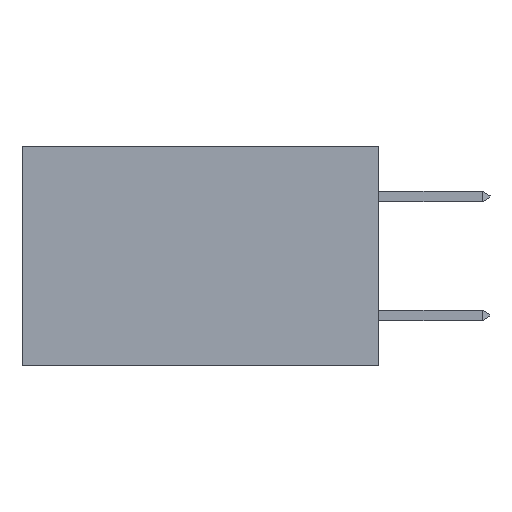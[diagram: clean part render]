
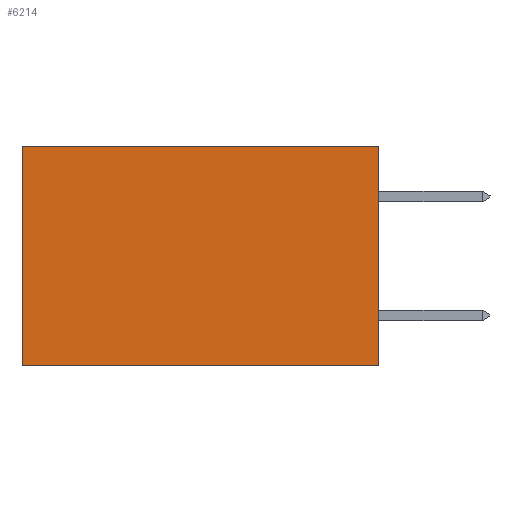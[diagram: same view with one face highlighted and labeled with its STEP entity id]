
A CAD part, left-side view. The second image highlights one B-rep face of the part: STEP entity #6214.
In plain terms, the highlighted planar face has unit normal (-1, 0, 0).
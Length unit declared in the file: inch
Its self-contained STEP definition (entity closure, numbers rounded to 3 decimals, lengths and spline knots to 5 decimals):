
#232 = DIRECTION ( 'NONE',  ( 0., 0., -1. ) ) ;
#414 = VERTEX_POINT ( 'NONE', #10315 ) ;
#859 = DIRECTION ( 'NONE',  ( 0., 1., 0. ) ) ;
#1289 = CARTESIAN_POINT ( 'NONE',  ( 0.2615, 0., 0. ) ) ;
#2617 = CARTESIAN_POINT ( 'NONE',  ( 0.2615, 0.6, -0.37 ) ) ;
#3015 = LINE ( 'NONE', #9256, #19265 ) ;
#3797 = AXIS2_PLACEMENT_3D ( 'NONE', #9443, #17130, #232 ) ;
#4141 = EDGE_CURVE ( 'NONE', #414, #11413, #12224, .T. ) ;
#4582 = EDGE_CURVE ( 'NONE', #12774, #414, #8636, .T. ) ;
#5208 = DIRECTION ( 'NONE',  ( 0., 0., -1. ) ) ;
#5294 = ORIENTED_EDGE ( 'NONE', *, *, #4582, .T. ) ;
#5436 = VECTOR ( 'NONE', #5208, 39.37008 ) ;
#5633 = ORIENTED_EDGE ( 'NONE', *, *, #19944, .F. ) ;
#5884 = DIRECTION ( 'NONE',  ( 0., 0., -1. ) ) ;
#5944 = VECTOR ( 'NONE', #859, 39.37008 ) ;
#6214 = ADVANCED_FACE ( 'NONE', ( #8006 ), #14265, .F. ) ;
#8006 = FACE_OUTER_BOUND ( 'NONE', #9538, .T. ) ;
#8281 = LINE ( 'NONE', #19129, #5436 ) ;
#8636 = LINE ( 'NONE', #19574, #5944 ) ;
#8800 = EDGE_CURVE ( 'NONE', #12774, #17832, #8281, .T. ) ;
#9256 = CARTESIAN_POINT ( 'NONE',  ( 0.2615, 0., -0.37 ) ) ;
#9443 = CARTESIAN_POINT ( 'NONE',  ( 0.2615, 0., -0.37 ) ) ;
#9538 = EDGE_LOOP ( 'NONE', ( #17155, #5633, #17065, #5294 ) ) ;
#10152 = CARTESIAN_POINT ( 'NONE',  ( 0.2615, 0., -0.37 ) ) ;
#10315 = CARTESIAN_POINT ( 'NONE',  ( 0.2615, 0.6, 0. ) ) ;
#11413 = VERTEX_POINT ( 'NONE', #14731 ) ;
#12224 = LINE ( 'NONE', #2617, #19367 ) ;
#12774 = VERTEX_POINT ( 'NONE', #1289 ) ;
#14075 = DIRECTION ( 'NONE',  ( 0., 1., 0. ) ) ;
#14265 = PLANE ( 'NONE',  #3797 ) ;
#14731 = CARTESIAN_POINT ( 'NONE',  ( 0.2615, 0.6, -0.37 ) ) ;
#17065 = ORIENTED_EDGE ( 'NONE', *, *, #8800, .F. ) ;
#17130 = DIRECTION ( 'NONE',  ( 1., 0., 0. ) ) ;
#17155 = ORIENTED_EDGE ( 'NONE', *, *, #4141, .T. ) ;
#17832 = VERTEX_POINT ( 'NONE', #10152 ) ;
#19129 = CARTESIAN_POINT ( 'NONE',  ( 0.2615, 0., -0.37 ) ) ;
#19265 = VECTOR ( 'NONE', #14075, 39.37008 ) ;
#19367 = VECTOR ( 'NONE', #5884, 39.37008 ) ;
#19574 = CARTESIAN_POINT ( 'NONE',  ( 0.2615, 0., 0. ) ) ;
#19944 = EDGE_CURVE ( 'NONE', #17832, #11413, #3015, .T. ) ;
